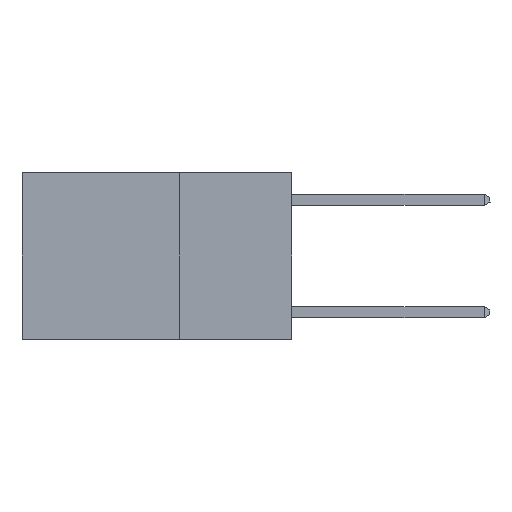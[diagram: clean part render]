
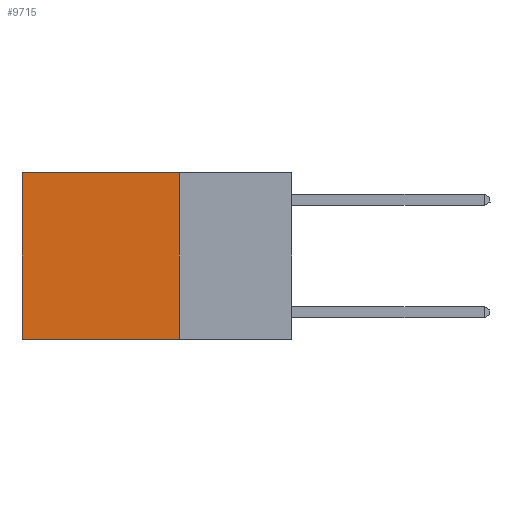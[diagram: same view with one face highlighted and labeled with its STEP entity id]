
A CAD part, left-side view. The second image highlights one B-rep face of the part: STEP entity #9715.
In plain terms, the highlighted planar face has unit normal (-1, 0, 0).
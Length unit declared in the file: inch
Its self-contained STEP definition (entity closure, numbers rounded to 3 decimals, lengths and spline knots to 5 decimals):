
#1232 = DIRECTION ( 'NONE',  ( 0., 0., -1. ) ) ;
#1899 = EDGE_CURVE ( 'NONE', #9854, #5120, #4687, .T. ) ;
#2700 = VECTOR ( 'NONE', #5698, 39.37008 ) ;
#2794 = EDGE_CURVE ( 'NONE', #9854, #5174, #2954, .T. ) ;
#2954 = LINE ( 'NONE', #4654, #4668 ) ;
#3019 = CARTESIAN_POINT ( 'NONE',  ( 0.2625, 0.6, 0. ) ) ;
#3220 = VECTOR ( 'NONE', #4093, 39.37008 ) ;
#3294 = VERTEX_POINT ( 'NONE', #9022 ) ;
#3448 = LINE ( 'NONE', #10329, #3220 ) ;
#3719 = CARTESIAN_POINT ( 'NONE',  ( 0.2625, 0.6, 0. ) ) ;
#3828 = LINE ( 'NONE', #3019, #9828 ) ;
#4093 = DIRECTION ( 'NONE',  ( 0., 1., 0. ) ) ;
#4403 = PLANE ( 'NONE',  #8584 ) ;
#4654 = CARTESIAN_POINT ( 'NONE',  ( 0.2625, 0.25, 0. ) ) ;
#4665 = CARTESIAN_POINT ( 'NONE',  ( 0.2625, 0.25, 0. ) ) ;
#4668 = VECTOR ( 'NONE', #6976, 39.37008 ) ;
#4678 = ORIENTED_EDGE ( 'NONE', *, *, #5220, .T. ) ;
#4687 = LINE ( 'NONE', #6668, #2700 ) ;
#4704 = ORIENTED_EDGE ( 'NONE', *, *, #6755, .F. ) ;
#4810 = ORIENTED_EDGE ( 'NONE', *, *, #1899, .F. ) ;
#4817 = ORIENTED_EDGE ( 'NONE', *, *, #2794, .T. ) ;
#5120 = VERTEX_POINT ( 'NONE', #6635 ) ;
#5174 = VERTEX_POINT ( 'NONE', #3719 ) ;
#5220 = EDGE_CURVE ( 'NONE', #5174, #3294, #3828, .T. ) ;
#5698 = DIRECTION ( 'NONE',  ( 0., 0., -1. ) ) ;
#5903 = DIRECTION ( 'NONE',  ( 1., 0., 0. ) ) ;
#6635 = CARTESIAN_POINT ( 'NONE',  ( 0.2625, 0.25, -0.37 ) ) ;
#6637 = CARTESIAN_POINT ( 'NONE',  ( 0.2625, 0.25, 0. ) ) ;
#6668 = CARTESIAN_POINT ( 'NONE',  ( 0.2625, 0.25, 0. ) ) ;
#6755 = EDGE_CURVE ( 'NONE', #5120, #3294, #3448, .T. ) ;
#6779 = FACE_OUTER_BOUND ( 'NONE', #7900, .T. ) ;
#6976 = DIRECTION ( 'NONE',  ( 0., 1., 0. ) ) ;
#7900 = EDGE_LOOP ( 'NONE', ( #4678, #4704, #4810, #4817 ) ) ;
#8584 = AXIS2_PLACEMENT_3D ( 'NONE', #6637, #5903, #1232 ) ;
#9022 = CARTESIAN_POINT ( 'NONE',  ( 0.2625, 0.6, -0.37 ) ) ;
#9715 = ADVANCED_FACE ( 'NONE', ( #6779 ), #4403, .F. ) ;
#9828 = VECTOR ( 'NONE', #10041, 39.37008 ) ;
#9854 = VERTEX_POINT ( 'NONE', #4665 ) ;
#10041 = DIRECTION ( 'NONE',  ( 0., 0., -1. ) ) ;
#10329 = CARTESIAN_POINT ( 'NONE',  ( 0.2625, 0.25, -0.37 ) ) ;
